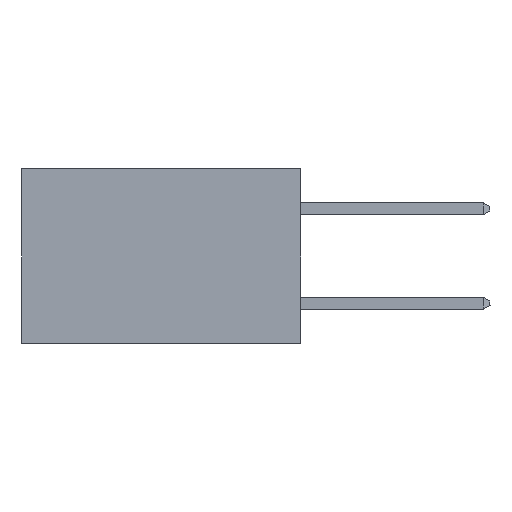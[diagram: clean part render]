
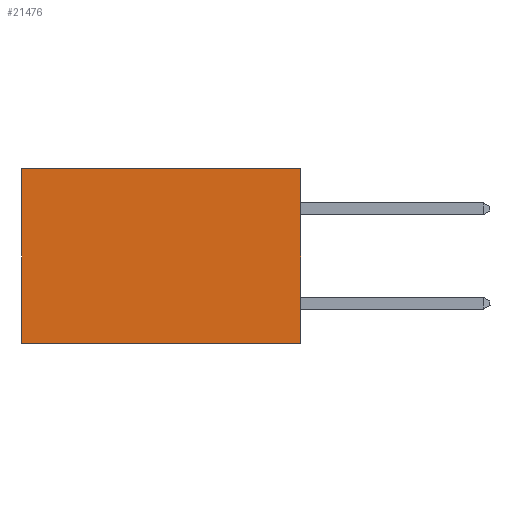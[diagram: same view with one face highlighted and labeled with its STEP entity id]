
A CAD part, left-side view. The second image highlights one B-rep face of the part: STEP entity #21476.
In plain terms, the highlighted planar face has unit normal (-1, 0, 0).
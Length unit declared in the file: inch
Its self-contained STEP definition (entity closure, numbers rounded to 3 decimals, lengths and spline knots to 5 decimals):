
#548 = ORIENTED_EDGE ( 'NONE', *, *, #2345, .F. ) ;
#631 = DIRECTION ( 'NONE',  ( 1., 0., 0. ) ) ;
#1127 = LINE ( 'NONE', #13589, #19099 ) ;
#1443 = VECTOR ( 'NONE', #5275, 39.37008 ) ;
#2345 = EDGE_CURVE ( 'NONE', #18965, #18484, #16545, .T. ) ;
#3312 = CARTESIAN_POINT ( 'NONE',  ( 0.277, 0., -0.37 ) ) ;
#3597 = CARTESIAN_POINT ( 'NONE',  ( 0.277, 0., -0.37 ) ) ;
#4140 = LINE ( 'NONE', #11940, #17485 ) ;
#4730 = EDGE_LOOP ( 'NONE', ( #7739, #20471, #548, #8153 ) ) ;
#4956 = DIRECTION ( 'NONE',  ( 0., 1., 0. ) ) ;
#5275 = DIRECTION ( 'NONE',  ( 0., 0., -1. ) ) ;
#6075 = LINE ( 'NONE', #8670, #1443 ) ;
#7739 = ORIENTED_EDGE ( 'NONE', *, *, #15846, .T. ) ;
#7840 = VECTOR ( 'NONE', #12481, 39.37008 ) ;
#8135 = VERTEX_POINT ( 'NONE', #16089 ) ;
#8153 = ORIENTED_EDGE ( 'NONE', *, *, #8404, .T. ) ;
#8404 = EDGE_CURVE ( 'NONE', #18965, #14463, #4140, .T. ) ;
#8670 = CARTESIAN_POINT ( 'NONE',  ( 0.277, 0.59, -0.37 ) ) ;
#9266 = PLANE ( 'NONE',  #16067 ) ;
#9867 = EDGE_CURVE ( 'NONE', #18484, #8135, #1127, .T. ) ;
#10386 = FACE_OUTER_BOUND ( 'NONE', #4730, .T. ) ;
#11394 = CARTESIAN_POINT ( 'NONE',  ( 0.277, 0., 0. ) ) ;
#11940 = CARTESIAN_POINT ( 'NONE',  ( 0.277, 0., 0. ) ) ;
#12294 = DIRECTION ( 'NONE',  ( 0., 1., 0. ) ) ;
#12481 = DIRECTION ( 'NONE',  ( 0., 0., -1. ) ) ;
#12745 = DIRECTION ( 'NONE',  ( 0., 0., -1. ) ) ;
#13589 = CARTESIAN_POINT ( 'NONE',  ( 0.277, 0., -0.37 ) ) ;
#14463 = VERTEX_POINT ( 'NONE', #16843 ) ;
#15846 = EDGE_CURVE ( 'NONE', #14463, #8135, #6075, .T. ) ;
#16067 = AXIS2_PLACEMENT_3D ( 'NONE', #21486, #631, #12745 ) ;
#16089 = CARTESIAN_POINT ( 'NONE',  ( 0.277, 0.59, -0.37 ) ) ;
#16545 = LINE ( 'NONE', #3597, #7840 ) ;
#16843 = CARTESIAN_POINT ( 'NONE',  ( 0.277, 0.59, 0. ) ) ;
#17485 = VECTOR ( 'NONE', #12294, 39.37008 ) ;
#18484 = VERTEX_POINT ( 'NONE', #3312 ) ;
#18965 = VERTEX_POINT ( 'NONE', #11394 ) ;
#19099 = VECTOR ( 'NONE', #4956, 39.37008 ) ;
#20471 = ORIENTED_EDGE ( 'NONE', *, *, #9867, .F. ) ;
#21476 = ADVANCED_FACE ( 'NONE', ( #10386 ), #9266, .F. ) ;
#21486 = CARTESIAN_POINT ( 'NONE',  ( 0.277, 0., -0.37 ) ) ;
